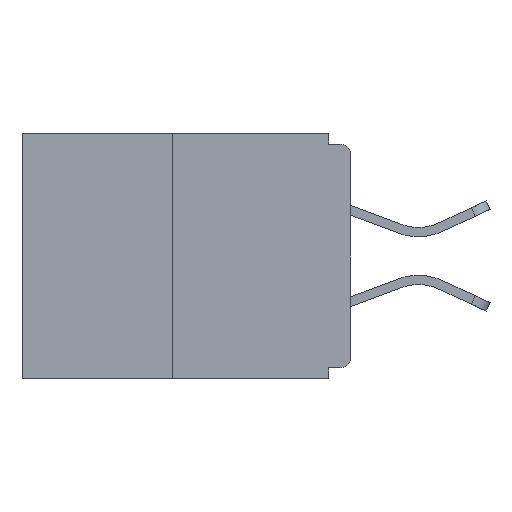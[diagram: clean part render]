
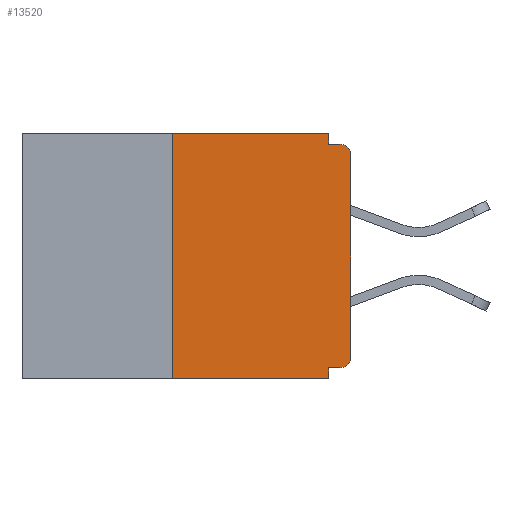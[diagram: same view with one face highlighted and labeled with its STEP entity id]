
A CAD part, left-side view. The second image highlights one B-rep face of the part: STEP entity #13520.
In plain terms, the highlighted planar face has unit normal (-1, 0, 0).
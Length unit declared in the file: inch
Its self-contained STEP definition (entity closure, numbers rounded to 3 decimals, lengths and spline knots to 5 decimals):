
#226 = VERTEX_POINT ( 'NONE', #19459 ) ;
#389 = CARTESIAN_POINT ( 'NONE',  ( 0., 0., 0. ) ) ;
#531 = LINE ( 'NONE', #17616, #17347 ) ;
#683 = VECTOR ( 'NONE', #29895, 39.37008 ) ;
#780 = DIRECTION ( 'NONE',  ( 0., -1., 0. ) ) ;
#1871 = LINE ( 'NONE', #27593, #683 ) ;
#2386 = AXIS2_PLACEMENT_3D ( 'NONE', #21907, #31911, #4300 ) ;
#2433 = LINE ( 'NONE', #18066, #28323 ) ;
#2516 = VERTEX_POINT ( 'NONE', #25711 ) ;
#2905 = CARTESIAN_POINT ( 'NONE',  ( 0., 0., -0.03 ) ) ;
#2908 = DIRECTION ( 'NONE',  ( 0., 0., 1. ) ) ;
#2999 = DIRECTION ( 'NONE',  ( 0., 0., 1. ) ) ;
#3560 = VERTEX_POINT ( 'NONE', #26099 ) ;
#3671 = ORIENTED_EDGE ( 'NONE', *, *, #28039, .F. ) ;
#4122 = ORIENTED_EDGE ( 'NONE', *, *, #32245, .T. ) ;
#4295 = CARTESIAN_POINT ( 'NONE',  ( 0., 0.031, -0.015 ) ) ;
#4300 = DIRECTION ( 'NONE',  ( 0., 0., -1. ) ) ;
#5051 = DIRECTION ( 'NONE',  ( 0., 0., -1. ) ) ;
#6084 = VERTEX_POINT ( 'NONE', #24561 ) ;
#7353 = PLANE ( 'NONE',  #22591 ) ;
#8667 = LINE ( 'NONE', #25635, #21924 ) ;
#8778 = LINE ( 'NONE', #15450, #13864 ) ;
#9120 = VECTOR ( 'NONE', #18019, 39.37008 ) ;
#9615 = CARTESIAN_POINT ( 'NONE',  ( 0., 0.25, -0.343 ) ) ;
#11268 = EDGE_CURVE ( 'NONE', #3560, #6084, #1871, .T. ) ;
#11306 = CARTESIAN_POINT ( 'NONE',  ( 0., 0.015, -0.03 ) ) ;
#11965 = ORIENTED_EDGE ( 'NONE', *, *, #27686, .F. ) ;
#12248 = ORIENTED_EDGE ( 'NONE', *, *, #20035, .F. ) ;
#12260 = DIRECTION ( 'NONE',  ( 1., 0., 0. ) ) ;
#12541 = CARTESIAN_POINT ( 'NONE',  ( 0., 0.25, 0. ) ) ;
#12784 = CARTESIAN_POINT ( 'NONE',  ( 0., 0.031, 0. ) ) ;
#13502 = LINE ( 'NONE', #389, #15840 ) ;
#13520 = ADVANCED_FACE ( 'NONE', ( #31082 ), #7353, .F. ) ;
#13585 = VERTEX_POINT ( 'NONE', #20856 ) ;
#13864 = VECTOR ( 'NONE', #5051, 39.37008 ) ;
#14426 = EDGE_CURVE ( 'NONE', #14984, #21174, #2433, .T. ) ;
#14984 = VERTEX_POINT ( 'NONE', #9615 ) ;
#15450 = CARTESIAN_POINT ( 'NONE',  ( 0., 0.031, 0. ) ) ;
#15741 = LINE ( 'NONE', #21777, #9120 ) ;
#15840 = VECTOR ( 'NONE', #2908, 39.37008 ) ;
#16213 = DIRECTION ( 'NONE',  ( -1., 0., 0. ) ) ;
#17038 = DIRECTION ( 'NONE',  ( 0., 0., -1. ) ) ;
#17347 = VECTOR ( 'NONE', #22577, 39.37008 ) ;
#17616 = CARTESIAN_POINT ( 'NONE',  ( 0., 0., -0.015 ) ) ;
#17831 = DIRECTION ( 'NONE',  ( 0., -1., 0. ) ) ;
#18019 = DIRECTION ( 'NONE',  ( 0., 0., -1. ) ) ;
#18066 = CARTESIAN_POINT ( 'NONE',  ( 0., 0.25, 0. ) ) ;
#18705 = DIRECTION ( 'NONE',  ( 0., 0., -1. ) ) ;
#18722 = ORIENTED_EDGE ( 'NONE', *, *, #28694, .T. ) ;
#19298 = AXIS2_PLACEMENT_3D ( 'NONE', #11306, #16213, #18705 ) ;
#19459 = CARTESIAN_POINT ( 'NONE',  ( 0., 0.015, -0.015 ) ) ;
#19981 = CARTESIAN_POINT ( 'NONE',  ( 0., 0.46, 0. ) ) ;
#20035 = EDGE_CURVE ( 'NONE', #21174, #26143, #27588, .T. ) ;
#20719 = CARTESIAN_POINT ( 'NONE',  ( 0., 0.46, 0. ) ) ;
#20856 = CARTESIAN_POINT ( 'NONE',  ( 0., 0.031, -0.343 ) ) ;
#21174 = VERTEX_POINT ( 'NONE', #12541 ) ;
#21743 = VERTEX_POINT ( 'NONE', #4295 ) ;
#21777 = CARTESIAN_POINT ( 'NONE',  ( 0., 0.031, -0.343 ) ) ;
#21907 = CARTESIAN_POINT ( 'NONE',  ( 0., 0.015, -0.313 ) ) ;
#21924 = VECTOR ( 'NONE', #17831, 39.37008 ) ;
#22577 = DIRECTION ( 'NONE',  ( 0., -1., 0. ) ) ;
#22591 = AXIS2_PLACEMENT_3D ( 'NONE', #19981, #12260, #17038 ) ;
#24387 = CIRCLE ( 'NONE', #19298, 0.015 ) ;
#24484 = ORIENTED_EDGE ( 'NONE', *, *, #29778, .T. ) ;
#24532 = ORIENTED_EDGE ( 'NONE', *, *, #14426, .F. ) ;
#24561 = CARTESIAN_POINT ( 'NONE',  ( 0., 0.031, -0.328 ) ) ;
#24844 = VECTOR ( 'NONE', #780, 39.37008 ) ;
#25635 = CARTESIAN_POINT ( 'NONE',  ( 0., 0.46, -0.343 ) ) ;
#25711 = CARTESIAN_POINT ( 'NONE',  ( 0., 0., -0.313 ) ) ;
#26099 = CARTESIAN_POINT ( 'NONE',  ( 0., 0.015, -0.328 ) ) ;
#26143 = VERTEX_POINT ( 'NONE', #12784 ) ;
#26164 = ORIENTED_EDGE ( 'NONE', *, *, #28787, .F. ) ;
#27422 = EDGE_CURVE ( 'NONE', #2516, #29096, #13502, .T. ) ;
#27588 = LINE ( 'NONE', #20719, #24844 ) ;
#27593 = CARTESIAN_POINT ( 'NONE',  ( 0., 0., -0.328 ) ) ;
#27686 = EDGE_CURVE ( 'NONE', #21743, #226, #531, .T. ) ;
#27939 = CIRCLE ( 'NONE', #2386, 0.015 ) ;
#28039 = EDGE_CURVE ( 'NONE', #26143, #21743, #8778, .T. ) ;
#28303 = EDGE_LOOP ( 'NONE', ( #12248, #24532, #24484, #26164, #29217, #4122, #32259, #18722, #11965, #3671 ) ) ;
#28323 = VECTOR ( 'NONE', #2999, 39.37008 ) ;
#28694 = EDGE_CURVE ( 'NONE', #29096, #226, #24387, .T. ) ;
#28787 = EDGE_CURVE ( 'NONE', #6084, #13585, #15741, .T. ) ;
#29096 = VERTEX_POINT ( 'NONE', #2905 ) ;
#29217 = ORIENTED_EDGE ( 'NONE', *, *, #11268, .F. ) ;
#29778 = EDGE_CURVE ( 'NONE', #14984, #13585, #8667, .T. ) ;
#29895 = DIRECTION ( 'NONE',  ( 0., 1., 0. ) ) ;
#31082 = FACE_OUTER_BOUND ( 'NONE', #28303, .T. ) ;
#31911 = DIRECTION ( 'NONE',  ( -1., 0., 0. ) ) ;
#32245 = EDGE_CURVE ( 'NONE', #3560, #2516, #27939, .T. ) ;
#32259 = ORIENTED_EDGE ( 'NONE', *, *, #27422, .T. ) ;
